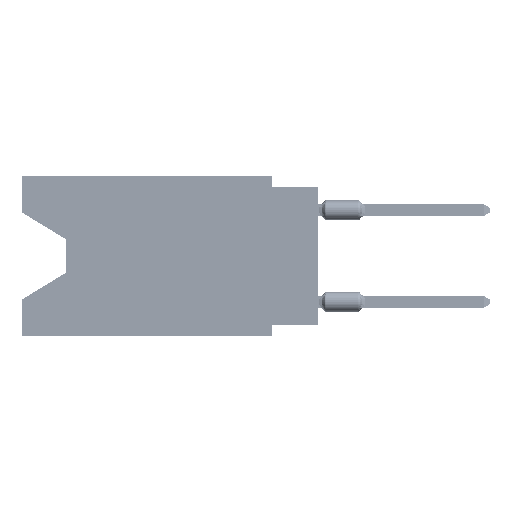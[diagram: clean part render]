
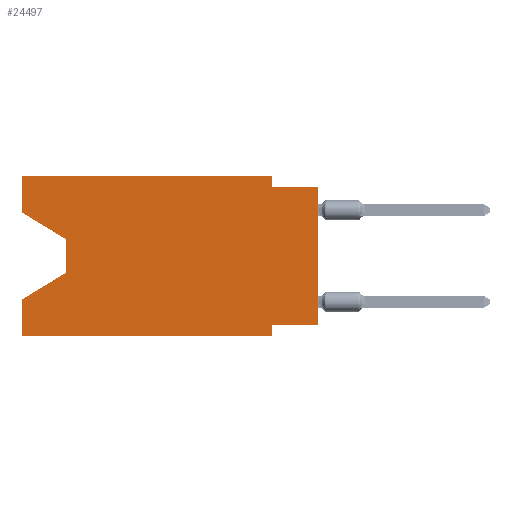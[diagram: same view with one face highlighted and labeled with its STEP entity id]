
A CAD part, left-side view. The second image highlights one B-rep face of the part: STEP entity #24497.
In plain terms, the highlighted planar face has unit normal (-1, 0, 0).
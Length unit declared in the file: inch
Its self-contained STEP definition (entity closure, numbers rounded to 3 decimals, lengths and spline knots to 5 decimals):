
#402 = CARTESIAN_POINT ( 'NONE',  ( 0., 0.645, 0. ) ) ;
#502 = VECTOR ( 'NONE', #3099, 39.37008 ) ;
#510 = LINE ( 'NONE', #70610, #5686 ) ;
#3099 = DIRECTION ( 'NONE',  ( 0., 1., 0. ) ) ;
#3904 = CARTESIAN_POINT ( 'NONE',  ( 0., 0.645, -0.08025 ) ) ;
#5302 = ORIENTED_EDGE ( 'NONE', *, *, #82506, .F. ) ;
#5686 = VECTOR ( 'NONE', #6597, 39.37008 ) ;
#5908 = LINE ( 'NONE', #62011, #16862 ) ;
#6597 = DIRECTION ( 'NONE',  ( 0., 0., -1. ) ) ;
#6895 = VERTEX_POINT ( 'NONE', #15279 ) ;
#8560 = VECTOR ( 'NONE', #42469, 39.37008 ) ;
#8670 = VECTOR ( 'NONE', #39324, 39.37008 ) ;
#9079 = VERTEX_POINT ( 'NONE', #61254 ) ;
#9657 = DIRECTION ( 'NONE',  ( 0., 0.855, -0.519 ) ) ;
#9905 = LINE ( 'NONE', #38413, #78860 ) ;
#10820 = CARTESIAN_POINT ( 'NONE',  ( 0., 0.55, -0.138 ) ) ;
#10918 = LINE ( 'NONE', #3904, #19579 ) ;
#12038 = VECTOR ( 'NONE', #9657, 39.37008 ) ;
#12095 = EDGE_CURVE ( 'NONE', #59122, #9079, #5908, .T. ) ;
#14412 = CARTESIAN_POINT ( 'NONE',  ( 0., 0.645, -0.26975 ) ) ;
#14916 = EDGE_CURVE ( 'NONE', #35487, #6895, #38625, .T. ) ;
#15279 = CARTESIAN_POINT ( 'NONE',  ( 0., 0.1, -0.325 ) ) ;
#16698 = CARTESIAN_POINT ( 'NONE',  ( 0., 0., -0.325 ) ) ;
#16862 = VECTOR ( 'NONE', #42347, 39.37008 ) ;
#17949 = VERTEX_POINT ( 'NONE', #14412 ) ;
#18685 = DIRECTION ( 'NONE',  ( 0., 0., -1. ) ) ;
#19579 = VECTOR ( 'NONE', #32395, 39.37008 ) ;
#19790 = CARTESIAN_POINT ( 'NONE',  ( 0., 0.55, -0.212 ) ) ;
#20179 = DIRECTION ( 'NONE',  ( 1., 0., 0. ) ) ;
#21268 = ORIENTED_EDGE ( 'NONE', *, *, #64536, .T. ) ;
#22480 = DIRECTION ( 'NONE',  ( 0., 0., 1. ) ) ;
#22853 = CARTESIAN_POINT ( 'NONE',  ( 0., 0., -0.025 ) ) ;
#24497 = ADVANCED_FACE ( 'NONE', ( #91658 ), #70126, .F. ) ;
#24625 = CARTESIAN_POINT ( 'NONE',  ( 0., 0.55, -0.212 ) ) ;
#24871 = CARTESIAN_POINT ( 'NONE',  ( 0., 0.645, 0. ) ) ;
#28777 = LINE ( 'NONE', #34397, #56555 ) ;
#29288 = ORIENTED_EDGE ( 'NONE', *, *, #69094, .F. ) ;
#32395 = DIRECTION ( 'NONE',  ( 0., -0.855, -0.519 ) ) ;
#32412 = VECTOR ( 'NONE', #46778, 39.37008 ) ;
#33310 = VERTEX_POINT ( 'NONE', #19790 ) ;
#34176 = VERTEX_POINT ( 'NONE', #64713 ) ;
#34397 = CARTESIAN_POINT ( 'NONE',  ( 0., 0., -0.025 ) ) ;
#34950 = CARTESIAN_POINT ( 'NONE',  ( 0., 0., -0.325 ) ) ;
#35487 = VERTEX_POINT ( 'NONE', #34950 ) ;
#38413 = CARTESIAN_POINT ( 'NONE',  ( 0., 0., 0. ) ) ;
#38625 = LINE ( 'NONE', #16698, #502 ) ;
#39324 = DIRECTION ( 'NONE',  ( 0., 0., -1. ) ) ;
#42347 = DIRECTION ( 'NONE',  ( 0., -1., 0. ) ) ;
#42469 = DIRECTION ( 'NONE',  ( 0., 0., 1. ) ) ;
#43958 = CARTESIAN_POINT ( 'NONE',  ( 0., 0.645, 0. ) ) ;
#45067 = CARTESIAN_POINT ( 'NONE',  ( 0., 0.645, -0.35 ) ) ;
#45606 = VERTEX_POINT ( 'NONE', #82262 ) ;
#46778 = DIRECTION ( 'NONE',  ( 0., -1., 0. ) ) ;
#48791 = ORIENTED_EDGE ( 'NONE', *, *, #56631, .F. ) ;
#50840 = ORIENTED_EDGE ( 'NONE', *, *, #60349, .F. ) ;
#51703 = LINE ( 'NONE', #24625, #12038 ) ;
#51946 = LINE ( 'NONE', #10820, #8670 ) ;
#53231 = LINE ( 'NONE', #90161, #57178 ) ;
#55486 = VECTOR ( 'NONE', #22480, 39.37008 ) ;
#56122 = DIRECTION ( 'NONE',  ( 0., 0., -1. ) ) ;
#56555 = VECTOR ( 'NONE', #63832, 39.37008 ) ;
#56631 = EDGE_CURVE ( 'NONE', #34176, #76539, #76681, .T. ) ;
#57178 = VECTOR ( 'NONE', #18685, 39.37008 ) ;
#57976 = EDGE_CURVE ( 'NONE', #45606, #33310, #51946, .T. ) ;
#58008 = EDGE_CURVE ( 'NONE', #35487, #75853, #9905, .T. ) ;
#59122 = VERTEX_POINT ( 'NONE', #45067 ) ;
#60349 = EDGE_CURVE ( 'NONE', #65640, #75853, #28777, .T. ) ;
#60748 = ORIENTED_EDGE ( 'NONE', *, *, #63939, .T. ) ;
#61254 = CARTESIAN_POINT ( 'NONE',  ( 0., 0.1, -0.35 ) ) ;
#61579 = VERTEX_POINT ( 'NONE', #74092 ) ;
#62011 = CARTESIAN_POINT ( 'NONE',  ( 0., 0.645, -0.35 ) ) ;
#63832 = DIRECTION ( 'NONE',  ( 0., -1., 0. ) ) ;
#63939 = EDGE_CURVE ( 'NONE', #33310, #17949, #51703, .T. ) ;
#64218 = ORIENTED_EDGE ( 'NONE', *, *, #58008, .T. ) ;
#64420 = LINE ( 'NONE', #402, #8560 ) ;
#64536 = EDGE_CURVE ( 'NONE', #61579, #45606, #10918, .T. ) ;
#64713 = CARTESIAN_POINT ( 'NONE',  ( 0., 0.645, 0. ) ) ;
#65640 = VERTEX_POINT ( 'NONE', #70045 ) ;
#69094 = EDGE_CURVE ( 'NONE', #76539, #65640, #53231, .T. ) ;
#70045 = CARTESIAN_POINT ( 'NONE',  ( 0., 0.1, -0.025 ) ) ;
#70126 = PLANE ( 'NONE',  #75891 ) ;
#70144 = LINE ( 'NONE', #43958, #55486 ) ;
#70610 = CARTESIAN_POINT ( 'NONE',  ( 0., 0.1, -0.35 ) ) ;
#72225 = ORIENTED_EDGE ( 'NONE', *, *, #14916, .F. ) ;
#72772 = ORIENTED_EDGE ( 'NONE', *, *, #57976, .T. ) ;
#74092 = CARTESIAN_POINT ( 'NONE',  ( 0., 0.645, -0.08025 ) ) ;
#75853 = VERTEX_POINT ( 'NONE', #22853 ) ;
#75891 = AXIS2_PLACEMENT_3D ( 'NONE', #77615, #20179, #56122 ) ;
#76539 = VERTEX_POINT ( 'NONE', #89506 ) ;
#76681 = LINE ( 'NONE', #24871, #32412 ) ;
#77615 = CARTESIAN_POINT ( 'NONE',  ( 0., 0.645, 0. ) ) ;
#78860 = VECTOR ( 'NONE', #88894, 39.37008 ) ;
#79214 = ORIENTED_EDGE ( 'NONE', *, *, #12095, .T. ) ;
#81335 = EDGE_LOOP ( 'NONE', ( #21268, #72772, #60748, #87005, #79214, #85845, #72225, #64218, #50840, #29288, #48791, #5302 ) ) ;
#82262 = CARTESIAN_POINT ( 'NONE',  ( 0., 0.55, -0.138 ) ) ;
#82506 = EDGE_CURVE ( 'NONE', #61579, #34176, #70144, .T. ) ;
#85845 = ORIENTED_EDGE ( 'NONE', *, *, #91665, .F. ) ;
#87005 = ORIENTED_EDGE ( 'NONE', *, *, #88855, .F. ) ;
#88855 = EDGE_CURVE ( 'NONE', #59122, #17949, #64420, .T. ) ;
#88894 = DIRECTION ( 'NONE',  ( 0., 0., 1. ) ) ;
#89506 = CARTESIAN_POINT ( 'NONE',  ( 0., 0.1, 0. ) ) ;
#90161 = CARTESIAN_POINT ( 'NONE',  ( 0., 0.1, 0. ) ) ;
#91658 = FACE_OUTER_BOUND ( 'NONE', #81335, .T. ) ;
#91665 = EDGE_CURVE ( 'NONE', #6895, #9079, #510, .T. ) ;
